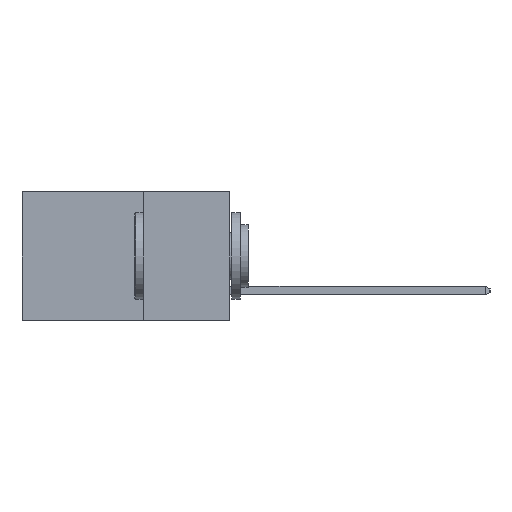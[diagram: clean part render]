
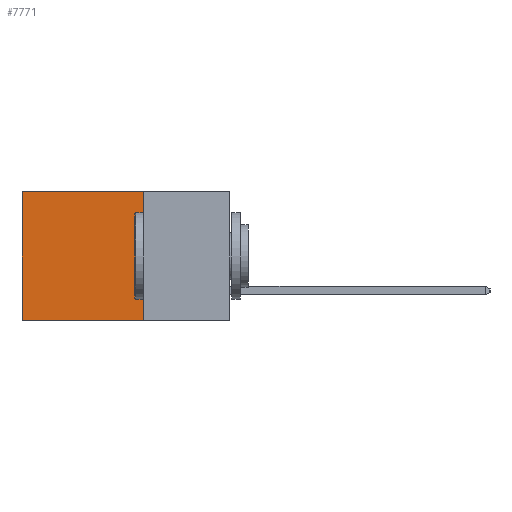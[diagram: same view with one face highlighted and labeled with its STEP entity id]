
A CAD part, left-side view. The second image highlights one B-rep face of the part: STEP entity #7771.
In plain terms, the highlighted planar face has unit normal (-1, 0, 0).
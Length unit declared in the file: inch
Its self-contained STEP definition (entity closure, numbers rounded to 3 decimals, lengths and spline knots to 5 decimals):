
#121 = CARTESIAN_POINT ( 'NONE',  ( 0.2615, 0.25, -0.37 ) ) ;
#2395 = VERTEX_POINT ( 'NONE', #121 ) ;
#2848 = VECTOR ( 'NONE', #16915, 39.37008 ) ;
#2872 = VECTOR ( 'NONE', #18747, 39.37008 ) ;
#3694 = CARTESIAN_POINT ( 'NONE',  ( 0.2615, 0.6, 0. ) ) ;
#4498 = VECTOR ( 'NONE', #13826, 39.37008 ) ;
#5029 = CARTESIAN_POINT ( 'NONE',  ( 0.2615, 0.25, -0.37 ) ) ;
#5315 = CARTESIAN_POINT ( 'NONE',  ( 0.2615, 0.25, 0. ) ) ;
#5727 = ORIENTED_EDGE ( 'NONE', *, *, #6922, .F. ) ;
#5958 = DIRECTION ( 'NONE',  ( 0., 0., -1. ) ) ;
#5980 = DIRECTION ( 'NONE',  ( 1., 0., 0. ) ) ;
#6011 = CARTESIAN_POINT ( 'NONE',  ( 0.2615, 0.25, -0.37 ) ) ;
#6102 = VERTEX_POINT ( 'NONE', #17910 ) ;
#6922 = EDGE_CURVE ( 'NONE', #2395, #6102, #9093, .T. ) ;
#6956 = LINE ( 'NONE', #18829, #2872 ) ;
#7384 = ORIENTED_EDGE ( 'NONE', *, *, #17908, .F. ) ;
#7635 = PLANE ( 'NONE',  #8526 ) ;
#7771 = ADVANCED_FACE ( 'NONE', ( #18131 ), #7635, .F. ) ;
#7978 = EDGE_CURVE ( 'NONE', #15536, #6102, #6956, .T. ) ;
#8526 = AXIS2_PLACEMENT_3D ( 'NONE', #6011, #5980, #5958 ) ;
#8541 = EDGE_LOOP ( 'NONE', ( #13854, #5727, #7384, #11594 ) ) ;
#8577 = LINE ( 'NONE', #5029, #4498 ) ;
#9093 = LINE ( 'NONE', #16844, #16206 ) ;
#9226 = VERTEX_POINT ( 'NONE', #12875 ) ;
#11594 = ORIENTED_EDGE ( 'NONE', *, *, #17422, .T. ) ;
#12875 = CARTESIAN_POINT ( 'NONE',  ( 0.2615, 0.25, 0. ) ) ;
#13826 = DIRECTION ( 'NONE',  ( 0., 0., -1. ) ) ;
#13854 = ORIENTED_EDGE ( 'NONE', *, *, #7978, .T. ) ;
#14613 = LINE ( 'NONE', #5315, #2848 ) ;
#15256 = DIRECTION ( 'NONE',  ( 0., 1., 0. ) ) ;
#15536 = VERTEX_POINT ( 'NONE', #3694 ) ;
#16206 = VECTOR ( 'NONE', #15256, 39.37008 ) ;
#16844 = CARTESIAN_POINT ( 'NONE',  ( 0.2615, 0.25, -0.37 ) ) ;
#16915 = DIRECTION ( 'NONE',  ( 0., 1., 0. ) ) ;
#17422 = EDGE_CURVE ( 'NONE', #9226, #15536, #14613, .T. ) ;
#17908 = EDGE_CURVE ( 'NONE', #9226, #2395, #8577, .T. ) ;
#17910 = CARTESIAN_POINT ( 'NONE',  ( 0.2615, 0.6, -0.37 ) ) ;
#18131 = FACE_OUTER_BOUND ( 'NONE', #8541, .T. ) ;
#18747 = DIRECTION ( 'NONE',  ( 0., 0., -1. ) ) ;
#18829 = CARTESIAN_POINT ( 'NONE',  ( 0.2615, 0.6, -0.37 ) ) ;
